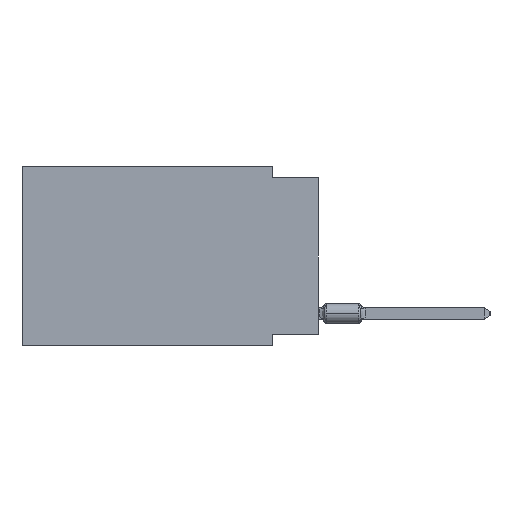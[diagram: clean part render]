
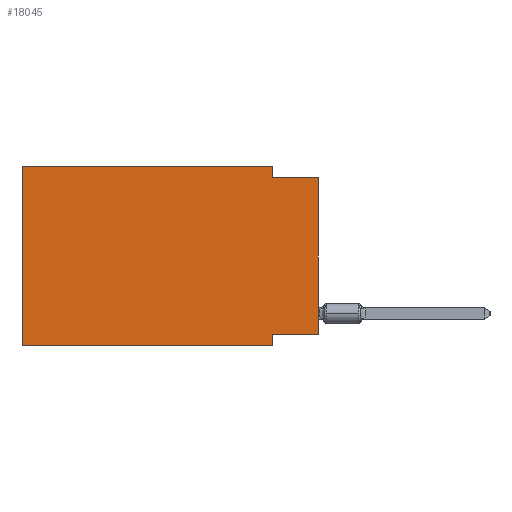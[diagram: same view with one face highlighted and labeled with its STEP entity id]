
A CAD part, left-side view. The second image highlights one B-rep face of the part: STEP entity #18045.
In plain terms, the highlighted planar face has unit normal (-1, 0, 0).
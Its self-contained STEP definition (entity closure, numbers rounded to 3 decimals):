
#1404 = CARTESIAN_POINT ( 'NONE',  ( 0., 16.383, 0. ) ) ;
#1701 = LINE ( 'NONE', #1404, #30957 ) ;
#2390 = CARTESIAN_POINT ( 'NONE',  ( 0., 0., 0. ) ) ;
#3789 = DIRECTION ( 'NONE',  ( 1., 0., 0. ) ) ;
#6826 = VECTOR ( 'NONE', #10539, 1000. ) ;
#7057 = VERTEX_POINT ( 'NONE', #57193 ) ;
#7190 = DIRECTION ( 'NONE',  ( 0., 0., 1. ) ) ;
#7583 = ORIENTED_EDGE ( 'NONE', *, *, #52211, .F. ) ;
#8016 = DIRECTION ( 'NONE',  ( 0., -1., 0. ) ) ;
#8945 = ORIENTED_EDGE ( 'NONE', *, *, #56037, .F. ) ;
#9077 = CARTESIAN_POINT ( 'NONE',  ( 0., 2.54, 0. ) ) ;
#10539 = DIRECTION ( 'NONE',  ( 0., 0., -1. ) ) ;
#11615 = ORIENTED_EDGE ( 'NONE', *, *, #57312, .T. ) ;
#11680 = DIRECTION ( 'NONE',  ( 0., -1., 0. ) ) ;
#12041 = VERTEX_POINT ( 'NONE', #25339 ) ;
#13312 = ORIENTED_EDGE ( 'NONE', *, *, #54844, .T. ) ;
#15227 = DIRECTION ( 'NONE',  ( 0., 0., 1. ) ) ;
#15947 = LINE ( 'NONE', #21019, #6826 ) ;
#16500 = LINE ( 'NONE', #2390, #48075 ) ;
#16810 = EDGE_LOOP ( 'NONE', ( #11615, #8945, #39564, #43439, #25095, #13312, #41457, #7583 ) ) ;
#18045 = ADVANCED_FACE ( 'NONE', ( #37130 ), #45817, .F. ) ;
#18273 = CARTESIAN_POINT ( 'NONE',  ( 0., 0., -9.271 ) ) ;
#21019 = CARTESIAN_POINT ( 'NONE',  ( 0., 2.54, 0. ) ) ;
#21981 = VECTOR ( 'NONE', #49422, 1000. ) ;
#24695 = CARTESIAN_POINT ( 'NONE',  ( 0., 2.54, -0.635 ) ) ;
#25095 = ORIENTED_EDGE ( 'NONE', *, *, #37981, .F. ) ;
#25229 = LINE ( 'NONE', #53672, #42176 ) ;
#25339 = CARTESIAN_POINT ( 'NONE',  ( 0., 16.383, 0. ) ) ;
#25661 = VERTEX_POINT ( 'NONE', #37631 ) ;
#26226 = DIRECTION ( 'NONE',  ( 0., 0., -1. ) ) ;
#27160 = VECTOR ( 'NONE', #26226, 1000. ) ;
#30812 = CARTESIAN_POINT ( 'NONE',  ( 0., 2.54, -9.271 ) ) ;
#30957 = VECTOR ( 'NONE', #15227, 1000. ) ;
#31150 = CARTESIAN_POINT ( 'NONE',  ( 0., 16.383, -9.906 ) ) ;
#31410 = VERTEX_POINT ( 'NONE', #35758 ) ;
#33816 = VERTEX_POINT ( 'NONE', #9077 ) ;
#34769 = LINE ( 'NONE', #31150, #21981 ) ;
#35758 = CARTESIAN_POINT ( 'NONE',  ( 0., 2.54, -9.906 ) ) ;
#36378 = LINE ( 'NONE', #53769, #46821 ) ;
#36849 = VERTEX_POINT ( 'NONE', #24695 ) ;
#37130 = FACE_OUTER_BOUND ( 'NONE', #16810, .T. ) ;
#37631 = CARTESIAN_POINT ( 'NONE',  ( 0., 16.383, -9.906 ) ) ;
#37981 = EDGE_CURVE ( 'NONE', #25661, #12041, #1701, .T. ) ;
#38858 = VERTEX_POINT ( 'NONE', #30812 ) ;
#39564 = ORIENTED_EDGE ( 'NONE', *, *, #42964, .F. ) ;
#39580 = LINE ( 'NONE', #49139, #56742 ) ;
#40004 = DIRECTION ( 'NONE',  ( 0., 1., 0. ) ) ;
#41457 = ORIENTED_EDGE ( 'NONE', *, *, #45020, .F. ) ;
#42176 = VECTOR ( 'NONE', #11680, 1000. ) ;
#42964 = EDGE_CURVE ( 'NONE', #33816, #36849, #15947, .T. ) ;
#43214 = AXIS2_PLACEMENT_3D ( 'NONE', #44936, #3789, #55389 ) ;
#43439 = ORIENTED_EDGE ( 'NONE', *, *, #43504, .F. ) ;
#43504 = EDGE_CURVE ( 'NONE', #12041, #33816, #39580, .T. ) ;
#44936 = CARTESIAN_POINT ( 'NONE',  ( 0., 16.383, 0. ) ) ;
#45020 = EDGE_CURVE ( 'NONE', #38858, #31410, #49294, .T. ) ;
#45817 = PLANE ( 'NONE',  #43214 ) ;
#46821 = VECTOR ( 'NONE', #40004, 1000. ) ;
#48075 = VECTOR ( 'NONE', #7190, 1000. ) ;
#49139 = CARTESIAN_POINT ( 'NONE',  ( 0., 16.383, 0. ) ) ;
#49294 = LINE ( 'NONE', #53492, #27160 ) ;
#49422 = DIRECTION ( 'NONE',  ( 0., -1., 0. ) ) ;
#51449 = VERTEX_POINT ( 'NONE', #18273 ) ;
#52211 = EDGE_CURVE ( 'NONE', #51449, #38858, #36378, .T. ) ;
#53492 = CARTESIAN_POINT ( 'NONE',  ( 0., 2.54, -9.906 ) ) ;
#53672 = CARTESIAN_POINT ( 'NONE',  ( 0., 0., -0.635 ) ) ;
#53769 = CARTESIAN_POINT ( 'NONE',  ( 0., 0., -9.271 ) ) ;
#54844 = EDGE_CURVE ( 'NONE', #25661, #31410, #34769, .T. ) ;
#55389 = DIRECTION ( 'NONE',  ( 0., 0., -1. ) ) ;
#56037 = EDGE_CURVE ( 'NONE', #36849, #7057, #25229, .T. ) ;
#56742 = VECTOR ( 'NONE', #8016, 1000. ) ;
#57193 = CARTESIAN_POINT ( 'NONE',  ( 0., 0., -0.635 ) ) ;
#57312 = EDGE_CURVE ( 'NONE', #51449, #7057, #16500, .T. ) ;
